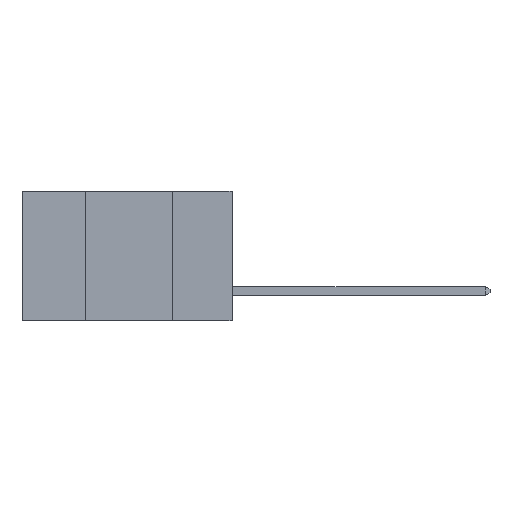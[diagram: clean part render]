
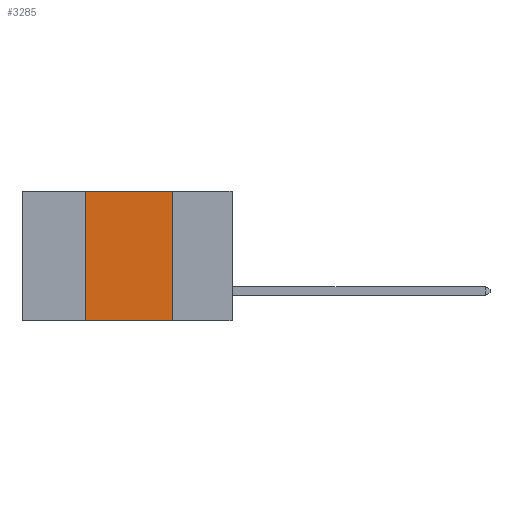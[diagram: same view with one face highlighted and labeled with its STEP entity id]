
A CAD part, left-side view. The second image highlights one B-rep face of the part: STEP entity #3285.
In plain terms, the highlighted planar face has unit normal (-1, 0, 0).
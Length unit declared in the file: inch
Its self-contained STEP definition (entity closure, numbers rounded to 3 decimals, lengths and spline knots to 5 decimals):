
#344 = LINE ( 'NONE', #1196, #5717 ) ;
#1196 = CARTESIAN_POINT ( 'NONE',  ( 0., 0.6, 0. ) ) ;
#2245 = VECTOR ( 'NONE', #21559, 39.37008 ) ;
#2845 = ORIENTED_EDGE ( 'NONE', *, *, #15352, .T. ) ;
#3285 = ADVANCED_FACE ( 'NONE', ( #8674 ), #3568, .F. ) ;
#3568 = PLANE ( 'NONE',  #18358 ) ;
#4464 = VECTOR ( 'NONE', #9888, 39.37008 ) ;
#4796 = VERTEX_POINT ( 'NONE', #16124 ) ;
#4867 = CARTESIAN_POINT ( 'NONE',  ( 0., 0.42, -0.37 ) ) ;
#5179 = LINE ( 'NONE', #7584, #4464 ) ;
#5717 = VECTOR ( 'NONE', #15027, 39.37008 ) ;
#7584 = CARTESIAN_POINT ( 'NONE',  ( 0., 0.6, -0.37 ) ) ;
#8157 = DIRECTION ( 'NONE',  ( 0., 0., -1. ) ) ;
#8674 = FACE_OUTER_BOUND ( 'NONE', #13705, .T. ) ;
#9522 = VERTEX_POINT ( 'NONE', #28659 ) ;
#9888 = DIRECTION ( 'NONE',  ( 0., -1., 0. ) ) ;
#10540 = ORIENTED_EDGE ( 'NONE', *, *, #11874, .F. ) ;
#11408 = LINE ( 'NONE', #22396, #16084 ) ;
#11874 = EDGE_CURVE ( 'NONE', #4796, #14189, #344, .T. ) ;
#12298 = ORIENTED_EDGE ( 'NONE', *, *, #13245, .F. ) ;
#13245 = EDGE_CURVE ( 'NONE', #14189, #9522, #11408, .T. ) ;
#13705 = EDGE_LOOP ( 'NONE', ( #12298, #10540, #14526, #2845 ) ) ;
#14189 = VERTEX_POINT ( 'NONE', #19091 ) ;
#14526 = ORIENTED_EDGE ( 'NONE', *, *, #29171, .F. ) ;
#15027 = DIRECTION ( 'NONE',  ( 0., -1., 0. ) ) ;
#15352 = EDGE_CURVE ( 'NONE', #27404, #9522, #5179, .T. ) ;
#16084 = VECTOR ( 'NONE', #24713, 39.37008 ) ;
#16124 = CARTESIAN_POINT ( 'NONE',  ( 0., 0.42, 0. ) ) ;
#18358 = AXIS2_PLACEMENT_3D ( 'NONE', #19595, #21899, #8157 ) ;
#19091 = CARTESIAN_POINT ( 'NONE',  ( 0., 0.17, 0. ) ) ;
#19595 = CARTESIAN_POINT ( 'NONE',  ( 0., 0.6, 0. ) ) ;
#21559 = DIRECTION ( 'NONE',  ( 0., 0., 1. ) ) ;
#21899 = DIRECTION ( 'NONE',  ( 1., 0., 0. ) ) ;
#22396 = CARTESIAN_POINT ( 'NONE',  ( 0., 0.17, 0. ) ) ;
#24713 = DIRECTION ( 'NONE',  ( 0., 0., -1. ) ) ;
#25990 = CARTESIAN_POINT ( 'NONE',  ( 0., 0.42, 0. ) ) ;
#26636 = LINE ( 'NONE', #25990, #2245 ) ;
#27404 = VERTEX_POINT ( 'NONE', #4867 ) ;
#28659 = CARTESIAN_POINT ( 'NONE',  ( 0., 0.17, -0.37 ) ) ;
#29171 = EDGE_CURVE ( 'NONE', #27404, #4796, #26636, .T. ) ;
